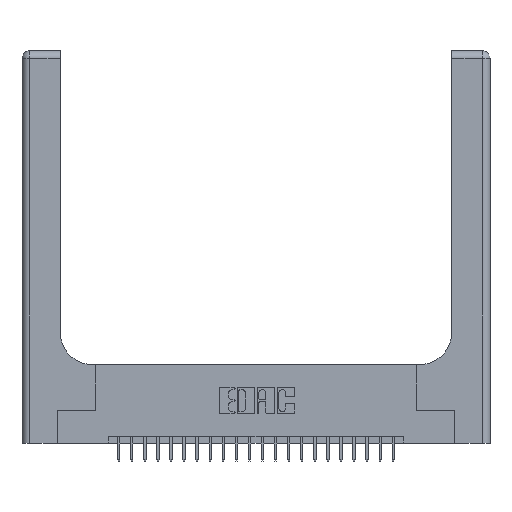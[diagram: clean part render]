
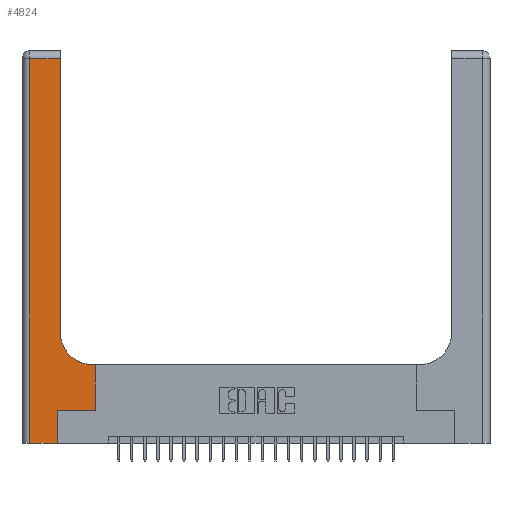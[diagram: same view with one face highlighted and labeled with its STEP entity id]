
A CAD part, top view. The second image highlights one B-rep face of the part: STEP entity #4824.
In plain terms, the highlighted planar face has unit normal (0, 0, 1).
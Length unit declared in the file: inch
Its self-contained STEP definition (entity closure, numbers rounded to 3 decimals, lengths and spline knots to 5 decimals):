
#517 = DIRECTION ( 'NONE',  ( -1., 0., 0. ) ) ;
#532 = VECTOR ( 'NONE', #15749, 39.37008 ) ;
#659 = VECTOR ( 'NONE', #7023, 39.37008 ) ;
#690 = DIRECTION ( 'NONE',  ( 1., 0., 0. ) ) ;
#1065 = LINE ( 'NONE', #14614, #3067 ) ;
#1689 = DIRECTION ( 'NONE',  ( 0., -1., 0. ) ) ;
#1966 = VECTOR ( 'NONE', #7893, 39.37008 ) ;
#2097 = LINE ( 'NONE', #7726, #6713 ) ;
#2199 = EDGE_CURVE ( 'NONE', #21038, #9376, #7690, .T. ) ;
#2445 = PLANE ( 'NONE',  #24628 ) ;
#3067 = VECTOR ( 'NONE', #690, 39.37008 ) ;
#3268 = CARTESIAN_POINT ( 'NONE',  ( 0., 0., 0.37 ) ) ;
#3329 = ORIENTED_EDGE ( 'NONE', *, *, #2199, .T. ) ;
#3640 = CARTESIAN_POINT ( 'NONE',  ( 0.06, 3., 0.37 ) ) ;
#3876 = EDGE_CURVE ( 'NONE', #14715, #24969, #2097, .T. ) ;
#3977 = CARTESIAN_POINT ( 'NONE',  ( 0.2915, 0.6, 0.37 ) ) ;
#4007 = CARTESIAN_POINT ( 'NONE',  ( 0., 3., 0.37 ) ) ;
#4824 = ADVANCED_FACE ( 'NONE', ( #9953 ), #2445, .F. ) ;
#5540 = ORIENTED_EDGE ( 'NONE', *, *, #22462, .T. ) ;
#6206 = EDGE_CURVE ( 'NONE', #24969, #12311, #1065, .T. ) ;
#6713 = VECTOR ( 'NONE', #13982, 39.37008 ) ;
#7023 = DIRECTION ( 'NONE',  ( -1., 0., 0. ) ) ;
#7474 = ORIENTED_EDGE ( 'NONE', *, *, #11457, .T. ) ;
#7690 = LINE ( 'NONE', #15502, #532 ) ;
#7726 = CARTESIAN_POINT ( 'NONE',  ( 0.269, 0., 0.37 ) ) ;
#7893 = DIRECTION ( 'NONE',  ( -1., 0., 0. ) ) ;
#9000 = CARTESIAN_POINT ( 'NONE',  ( 0.269, 0.25, 0.37 ) ) ;
#9004 = LINE ( 'NONE', #10410, #19790 ) ;
#9376 = VERTEX_POINT ( 'NONE', #23661 ) ;
#9953 = FACE_OUTER_BOUND ( 'NONE', #18051, .T. ) ;
#10223 = DIRECTION ( 'NONE',  ( 0., 0., -1. ) ) ;
#10410 = CARTESIAN_POINT ( 'NONE',  ( 0.5585, 0.25, 0.37 ) ) ;
#10451 = ORIENTED_EDGE ( 'NONE', *, *, #22195, .T. ) ;
#10602 = EDGE_CURVE ( 'NONE', #23818, #18056, #21476, .T. ) ;
#10660 = DIRECTION ( 'NONE',  ( 1., 0., 0. ) ) ;
#11155 = LINE ( 'NONE', #3268, #11757 ) ;
#11457 = EDGE_CURVE ( 'NONE', #9376, #16709, #17142, .T. ) ;
#11757 = VECTOR ( 'NONE', #24699, 39.37008 ) ;
#12261 = CARTESIAN_POINT ( 'NONE',  ( 0.06, 2.94, 0.37 ) ) ;
#12311 = VERTEX_POINT ( 'NONE', #21210 ) ;
#12430 = CARTESIAN_POINT ( 'NONE',  ( 0.5415, 0.6, 0.37 ) ) ;
#12803 = CARTESIAN_POINT ( 'NONE',  ( 0.2915, 0.85, 0.37 ) ) ;
#12830 = EDGE_CURVE ( 'NONE', #16709, #16924, #13306, .T. ) ;
#13306 = LINE ( 'NONE', #3640, #21315 ) ;
#13982 = DIRECTION ( 'NONE',  ( 0., 1., 0. ) ) ;
#14370 = DIRECTION ( 'NONE',  ( 0., 0., -1. ) ) ;
#14614 = CARTESIAN_POINT ( 'NONE',  ( 0.269, 0.25, 0.37 ) ) ;
#14715 = VERTEX_POINT ( 'NONE', #22887 ) ;
#15092 = CARTESIAN_POINT ( 'NONE',  ( 0.06, 0., 0.37 ) ) ;
#15502 = CARTESIAN_POINT ( 'NONE',  ( 0.2915, 3., 0.37 ) ) ;
#15749 = DIRECTION ( 'NONE',  ( 0., 1., 0. ) ) ;
#15943 = EDGE_CURVE ( 'NONE', #12311, #23818, #9004, .T. ) ;
#16353 = ORIENTED_EDGE ( 'NONE', *, *, #15943, .T. ) ;
#16703 = ORIENTED_EDGE ( 'NONE', *, *, #12830, .T. ) ;
#16709 = VERTEX_POINT ( 'NONE', #12261 ) ;
#16833 = ORIENTED_EDGE ( 'NONE', *, *, #3876, .T. ) ;
#16924 = VERTEX_POINT ( 'NONE', #15092 ) ;
#17142 = LINE ( 'NONE', #24657, #659 ) ;
#17311 = CARTESIAN_POINT ( 'NONE',  ( 0.5585, 0.6, 0.37 ) ) ;
#18051 = EDGE_LOOP ( 'NONE', ( #3329, #7474, #16703, #5540, #16833, #21849, #16353, #23653, #10451 ) ) ;
#18056 = VERTEX_POINT ( 'NONE', #12430 ) ;
#18288 = CIRCLE ( 'NONE', #21571, 0.25 ) ;
#18366 = DIRECTION ( 'NONE',  ( 0., 1., 0. ) ) ;
#18475 = CARTESIAN_POINT ( 'NONE',  ( 0.5415, 0.85, 0.37 ) ) ;
#19790 = VECTOR ( 'NONE', #18366, 39.37008 ) ;
#21038 = VERTEX_POINT ( 'NONE', #12803 ) ;
#21210 = CARTESIAN_POINT ( 'NONE',  ( 0.5585, 0.25, 0.37 ) ) ;
#21315 = VECTOR ( 'NONE', #1689, 39.37008 ) ;
#21476 = LINE ( 'NONE', #3977, #1966 ) ;
#21571 = AXIS2_PLACEMENT_3D ( 'NONE', #18475, #14370, #10660 ) ;
#21849 = ORIENTED_EDGE ( 'NONE', *, *, #6206, .T. ) ;
#22195 = EDGE_CURVE ( 'NONE', #18056, #21038, #18288, .T. ) ;
#22462 = EDGE_CURVE ( 'NONE', #16924, #14715, #11155, .T. ) ;
#22887 = CARTESIAN_POINT ( 'NONE',  ( 0.269, 0., 0.37 ) ) ;
#23653 = ORIENTED_EDGE ( 'NONE', *, *, #10602, .T. ) ;
#23661 = CARTESIAN_POINT ( 'NONE',  ( 0.2915, 2.94, 0.37 ) ) ;
#23818 = VERTEX_POINT ( 'NONE', #17311 ) ;
#24628 = AXIS2_PLACEMENT_3D ( 'NONE', #4007, #10223, #517 ) ;
#24657 = CARTESIAN_POINT ( 'NONE',  ( 0., 2.94, 0.37 ) ) ;
#24699 = DIRECTION ( 'NONE',  ( 1., 0., 0. ) ) ;
#24969 = VERTEX_POINT ( 'NONE', #9000 ) ;
